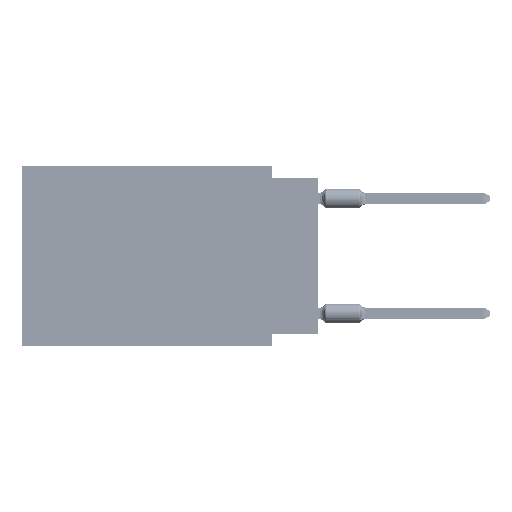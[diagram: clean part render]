
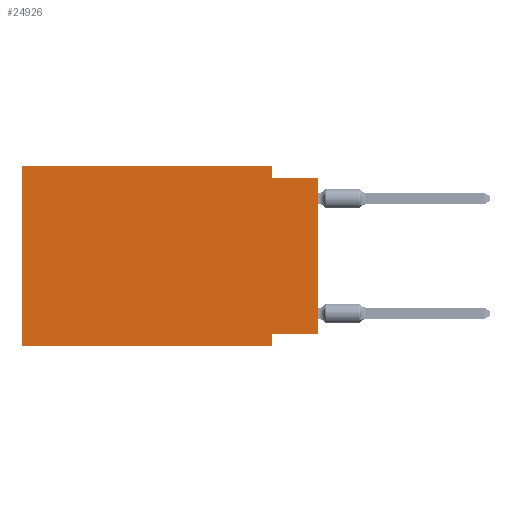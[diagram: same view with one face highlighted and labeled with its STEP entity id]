
A CAD part, left-side view. The second image highlights one B-rep face of the part: STEP entity #24926.
In plain terms, the highlighted planar face has unit normal (-1, 0, 0).
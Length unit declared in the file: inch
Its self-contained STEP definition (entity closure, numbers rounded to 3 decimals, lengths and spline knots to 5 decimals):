
#1943 = CARTESIAN_POINT ( 'NONE',  ( 0., 0.645, 0. ) ) ;
#3131 = DIRECTION ( 'NONE',  ( 0., 0., -1. ) ) ;
#3607 = LINE ( 'NONE', #48697, #22646 ) ;
#7161 = CARTESIAN_POINT ( 'NONE',  ( 0., 0.1, -0.365 ) ) ;
#7462 = ORIENTED_EDGE ( 'NONE', *, *, #70150, .T. ) ;
#7569 = EDGE_CURVE ( 'NONE', #15250, #53822, #26434, .T. ) ;
#13082 = ORIENTED_EDGE ( 'NONE', *, *, #7569, .T. ) ;
#14880 = CARTESIAN_POINT ( 'NONE',  ( 0., 0., -0.365 ) ) ;
#15250 = VERTEX_POINT ( 'NONE', #69021 ) ;
#15315 = CARTESIAN_POINT ( 'NONE',  ( 0., 0.1, 0. ) ) ;
#16329 = CARTESIAN_POINT ( 'NONE',  ( 0., 0.645, 0. ) ) ;
#18711 = DIRECTION ( 'NONE',  ( 0., -1., 0. ) ) ;
#19106 = CARTESIAN_POINT ( 'NONE',  ( 0., 0.645, -0.39 ) ) ;
#19239 = VECTOR ( 'NONE', #20599, 39.37008 ) ;
#19750 = ORIENTED_EDGE ( 'NONE', *, *, #79177, .F. ) ;
#20599 = DIRECTION ( 'NONE',  ( 0., -1., 0. ) ) ;
#21091 = VERTEX_POINT ( 'NONE', #49442 ) ;
#21125 = VECTOR ( 'NONE', #18711, 39.37008 ) ;
#21391 = VERTEX_POINT ( 'NONE', #59513 ) ;
#22423 = FACE_OUTER_BOUND ( 'NONE', #70772, .T. ) ;
#22646 = VECTOR ( 'NONE', #53568, 39.37008 ) ;
#24926 = ADVANCED_FACE ( 'NONE', ( #22423 ), #48016, .F. ) ;
#26434 = LINE ( 'NONE', #19106, #21125 ) ;
#26591 = VECTOR ( 'NONE', #68548, 39.37008 ) ;
#27918 = LINE ( 'NONE', #15315, #35685 ) ;
#31687 = VECTOR ( 'NONE', #75266, 39.37008 ) ;
#35669 = DIRECTION ( 'NONE',  ( 0., 0., -1. ) ) ;
#35685 = VECTOR ( 'NONE', #3131, 39.37008 ) ;
#35986 = ORIENTED_EDGE ( 'NONE', *, *, #38697, .F. ) ;
#36766 = CARTESIAN_POINT ( 'NONE',  ( 0., 0., -0.025 ) ) ;
#37204 = VERTEX_POINT ( 'NONE', #53003 ) ;
#37554 = CARTESIAN_POINT ( 'NONE',  ( 0., 0.1, -0.39 ) ) ;
#38339 = LINE ( 'NONE', #45633, #31687 ) ;
#38697 = EDGE_CURVE ( 'NONE', #15250, #21391, #38339, .T. ) ;
#40073 = LINE ( 'NONE', #14880, #62968 ) ;
#41130 = DIRECTION ( 'NONE',  ( 0., 0., -1. ) ) ;
#42809 = VERTEX_POINT ( 'NONE', #75555 ) ;
#43732 = ORIENTED_EDGE ( 'NONE', *, *, #67131, .F. ) ;
#45633 = CARTESIAN_POINT ( 'NONE',  ( 0., 0.645, 0. ) ) ;
#46346 = VERTEX_POINT ( 'NONE', #7161 ) ;
#48016 = PLANE ( 'NONE',  #66856 ) ;
#48697 = CARTESIAN_POINT ( 'NONE',  ( 0., 0., 0. ) ) ;
#49442 = CARTESIAN_POINT ( 'NONE',  ( 0., 0.1, 0. ) ) ;
#51759 = VERTEX_POINT ( 'NONE', #36766 ) ;
#53003 = CARTESIAN_POINT ( 'NONE',  ( 0., 0.1, -0.025 ) ) ;
#53568 = DIRECTION ( 'NONE',  ( 0., 0., 1. ) ) ;
#53822 = VERTEX_POINT ( 'NONE', #63653 ) ;
#57310 = EDGE_CURVE ( 'NONE', #46346, #53822, #68811, .T. ) ;
#59513 = CARTESIAN_POINT ( 'NONE',  ( 0., 0.645, 0. ) ) ;
#60867 = ORIENTED_EDGE ( 'NONE', *, *, #67659, .F. ) ;
#62968 = VECTOR ( 'NONE', #65635, 39.37008 ) ;
#63653 = CARTESIAN_POINT ( 'NONE',  ( 0., 0.1, -0.39 ) ) ;
#65614 = ORIENTED_EDGE ( 'NONE', *, *, #67040, .F. ) ;
#65635 = DIRECTION ( 'NONE',  ( 0., 1., 0. ) ) ;
#65666 = LINE ( 'NONE', #76212, #19239 ) ;
#66856 = AXIS2_PLACEMENT_3D ( 'NONE', #16329, #71552, #41130 ) ;
#67040 = EDGE_CURVE ( 'NONE', #21391, #21091, #75021, .T. ) ;
#67131 = EDGE_CURVE ( 'NONE', #21091, #37204, #27918, .T. ) ;
#67659 = EDGE_CURVE ( 'NONE', #42809, #46346, #40073, .T. ) ;
#68548 = DIRECTION ( 'NONE',  ( 0., -1., 0. ) ) ;
#68719 = VECTOR ( 'NONE', #35669, 39.37008 ) ;
#68811 = LINE ( 'NONE', #37554, #68719 ) ;
#69021 = CARTESIAN_POINT ( 'NONE',  ( 0., 0.645, -0.39 ) ) ;
#70150 = EDGE_CURVE ( 'NONE', #42809, #51759, #3607, .T. ) ;
#70772 = EDGE_LOOP ( 'NONE', ( #7462, #19750, #43732, #65614, #35986, #13082, #71321, #60867 ) ) ;
#71321 = ORIENTED_EDGE ( 'NONE', *, *, #57310, .F. ) ;
#71552 = DIRECTION ( 'NONE',  ( 1., 0., 0. ) ) ;
#75021 = LINE ( 'NONE', #1943, #26591 ) ;
#75266 = DIRECTION ( 'NONE',  ( 0., 0., 1. ) ) ;
#75555 = CARTESIAN_POINT ( 'NONE',  ( 0., 0., -0.365 ) ) ;
#76212 = CARTESIAN_POINT ( 'NONE',  ( 0., 0., -0.025 ) ) ;
#79177 = EDGE_CURVE ( 'NONE', #37204, #51759, #65666, .T. ) ;
